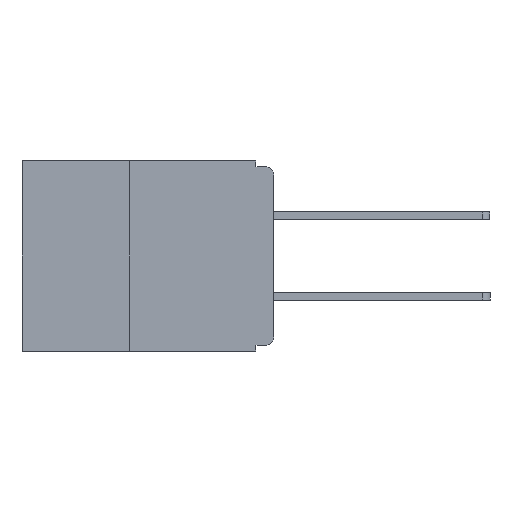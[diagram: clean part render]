
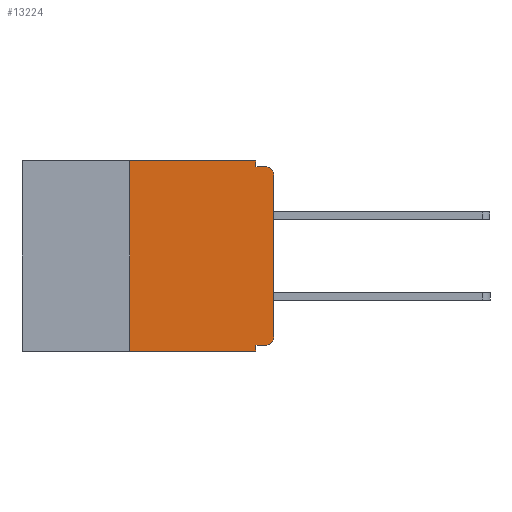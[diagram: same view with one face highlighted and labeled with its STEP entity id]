
A CAD part, left-side view. The second image highlights one B-rep face of the part: STEP entity #13224.
In plain terms, the highlighted planar face has unit normal (-1, 0, 0).
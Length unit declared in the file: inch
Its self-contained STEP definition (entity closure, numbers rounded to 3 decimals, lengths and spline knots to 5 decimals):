
#36 = LINE ( 'NONE', #5544, #14230 ) ;
#39 = LINE ( 'NONE', #6742, #3325 ) ;
#58 = DIRECTION ( 'NONE',  ( 0., -1., 0. ) ) ;
#118 = CARTESIAN_POINT ( 'NONE',  ( 0., 0.015, -0.32 ) ) ;
#161 = ORIENTED_EDGE ( 'NONE', *, *, #8990, .F. ) ;
#501 = EDGE_CURVE ( 'NONE', #9262, #522, #36, .T. ) ;
#522 = VERTEX_POINT ( 'NONE', #10559 ) ;
#686 = EDGE_LOOP ( 'NONE', ( #8285, #3920, #4875, #161, #5213, #11340, #8203, #12190, #4946, #6092 ) ) ;
#957 = DIRECTION ( 'NONE',  ( -1., 0., 0. ) ) ;
#1007 = CARTESIAN_POINT ( 'NONE',  ( 0., 0., -0.305 ) ) ;
#1153 = VERTEX_POINT ( 'NONE', #4699 ) ;
#1294 = DIRECTION ( 'NONE',  ( -1., 0., 0. ) ) ;
#1318 = VERTEX_POINT ( 'NONE', #16047 ) ;
#1646 = CARTESIAN_POINT ( 'NONE',  ( 0., 0.437, 0. ) ) ;
#1673 = VECTOR ( 'NONE', #8402, 39.37008 ) ;
#1788 = DIRECTION ( 'NONE',  ( 0., 0., 1. ) ) ;
#2535 = EDGE_CURVE ( 'NONE', #7679, #8561, #12140, .T. ) ;
#2536 = LINE ( 'NONE', #1646, #6807 ) ;
#2817 = VECTOR ( 'NONE', #12300, 39.37008 ) ;
#3325 = VECTOR ( 'NONE', #5270, 39.37008 ) ;
#3413 = VERTEX_POINT ( 'NONE', #15388 ) ;
#3920 = ORIENTED_EDGE ( 'NONE', *, *, #10655, .T. ) ;
#4338 = LINE ( 'NONE', #6071, #11266 ) ;
#4404 = DIRECTION ( 'NONE',  ( 0., -1., 0. ) ) ;
#4699 = CARTESIAN_POINT ( 'NONE',  ( 0., 0.25, 0. ) ) ;
#4875 = ORIENTED_EDGE ( 'NONE', *, *, #12992, .F. ) ;
#4946 = ORIENTED_EDGE ( 'NONE', *, *, #8838, .F. ) ;
#4962 = CARTESIAN_POINT ( 'NONE',  ( 0., 0., -0.32 ) ) ;
#5213 = ORIENTED_EDGE ( 'NONE', *, *, #6854, .F. ) ;
#5270 = DIRECTION ( 'NONE',  ( 0., 0., -1. ) ) ;
#5429 = LINE ( 'NONE', #5582, #1673 ) ;
#5544 = CARTESIAN_POINT ( 'NONE',  ( 0., 0.437, -0.33 ) ) ;
#5582 = CARTESIAN_POINT ( 'NONE',  ( 0., 0., -0.01 ) ) ;
#5583 = VECTOR ( 'NONE', #15745, 39.37008 ) ;
#6071 = CARTESIAN_POINT ( 'NONE',  ( 0., 0.25, -0.33 ) ) ;
#6092 = ORIENTED_EDGE ( 'NONE', *, *, #16245, .T. ) ;
#6152 = DIRECTION ( 'NONE',  ( 1., 0., 0. ) ) ;
#6241 = EDGE_CURVE ( 'NONE', #9262, #1153, #4338, .T. ) ;
#6742 = CARTESIAN_POINT ( 'NONE',  ( 0., 0.031, 0. ) ) ;
#6807 = VECTOR ( 'NONE', #4404, 39.37008 ) ;
#6854 = EDGE_CURVE ( 'NONE', #1153, #7170, #2536, .T. ) ;
#6871 = VERTEX_POINT ( 'NONE', #15308 ) ;
#7169 = AXIS2_PLACEMENT_3D ( 'NONE', #10213, #6152, #15501 ) ;
#7170 = VERTEX_POINT ( 'NONE', #8238 ) ;
#7679 = VERTEX_POINT ( 'NONE', #1007 ) ;
#8203 = ORIENTED_EDGE ( 'NONE', *, *, #501, .T. ) ;
#8238 = CARTESIAN_POINT ( 'NONE',  ( 0., 0.031, 0. ) ) ;
#8285 = ORIENTED_EDGE ( 'NONE', *, *, #2535, .T. ) ;
#8402 = DIRECTION ( 'NONE',  ( 0., -1., 0. ) ) ;
#8561 = VERTEX_POINT ( 'NONE', #11196 ) ;
#8773 = CIRCLE ( 'NONE', #9280, 0.015 ) ;
#8838 = EDGE_CURVE ( 'NONE', #13075, #1318, #13240, .T. ) ;
#8846 = PLANE ( 'NONE',  #7169 ) ;
#8883 = AXIS2_PLACEMENT_3D ( 'NONE', #9658, #1294, #11021 ) ;
#8990 = EDGE_CURVE ( 'NONE', #7170, #6871, #39, .T. ) ;
#9262 = VERTEX_POINT ( 'NONE', #15613 ) ;
#9280 = AXIS2_PLACEMENT_3D ( 'NONE', #9340, #957, #10705 ) ;
#9340 = CARTESIAN_POINT ( 'NONE',  ( 0., 0.015, -0.025 ) ) ;
#9455 = LINE ( 'NONE', #15998, #16037 ) ;
#9658 = CARTESIAN_POINT ( 'NONE',  ( 0., 0.015, -0.305 ) ) ;
#10213 = CARTESIAN_POINT ( 'NONE',  ( 0., 0.437, 0. ) ) ;
#10559 = CARTESIAN_POINT ( 'NONE',  ( 0., 0.031, -0.33 ) ) ;
#10655 = EDGE_CURVE ( 'NONE', #8561, #3413, #8773, .T. ) ;
#10705 = DIRECTION ( 'NONE',  ( 0., 0., -1. ) ) ;
#10810 = DIRECTION ( 'NONE',  ( 0., 0., -1. ) ) ;
#11021 = DIRECTION ( 'NONE',  ( 0., 0., -1. ) ) ;
#11196 = CARTESIAN_POINT ( 'NONE',  ( 0., 0., -0.025 ) ) ;
#11266 = VECTOR ( 'NONE', #1788, 39.37008 ) ;
#11340 = ORIENTED_EDGE ( 'NONE', *, *, #6241, .F. ) ;
#12140 = LINE ( 'NONE', #12181, #2817 ) ;
#12181 = CARTESIAN_POINT ( 'NONE',  ( 0., 0., 0. ) ) ;
#12190 = ORIENTED_EDGE ( 'NONE', *, *, #15522, .F. ) ;
#12300 = DIRECTION ( 'NONE',  ( 0., 0., 1. ) ) ;
#12489 = FACE_OUTER_BOUND ( 'NONE', #686, .T. ) ;
#12992 = EDGE_CURVE ( 'NONE', #6871, #3413, #5429, .T. ) ;
#13005 = CIRCLE ( 'NONE', #8883, 0.015 ) ;
#13075 = VERTEX_POINT ( 'NONE', #118 ) ;
#13224 = ADVANCED_FACE ( 'NONE', ( #12489 ), #8846, .F. ) ;
#13240 = LINE ( 'NONE', #4962, #5583 ) ;
#14230 = VECTOR ( 'NONE', #58, 39.37008 ) ;
#15308 = CARTESIAN_POINT ( 'NONE',  ( 0., 0.031, -0.01 ) ) ;
#15388 = CARTESIAN_POINT ( 'NONE',  ( 0., 0.015, -0.01 ) ) ;
#15501 = DIRECTION ( 'NONE',  ( 0., 0., -1. ) ) ;
#15522 = EDGE_CURVE ( 'NONE', #1318, #522, #9455, .T. ) ;
#15613 = CARTESIAN_POINT ( 'NONE',  ( 0., 0.25, -0.33 ) ) ;
#15745 = DIRECTION ( 'NONE',  ( 0., 1., 0. ) ) ;
#15998 = CARTESIAN_POINT ( 'NONE',  ( 0., 0.031, -0.33 ) ) ;
#16037 = VECTOR ( 'NONE', #10810, 39.37008 ) ;
#16047 = CARTESIAN_POINT ( 'NONE',  ( 0., 0.031, -0.32 ) ) ;
#16245 = EDGE_CURVE ( 'NONE', #13075, #7679, #13005, .T. ) ;
